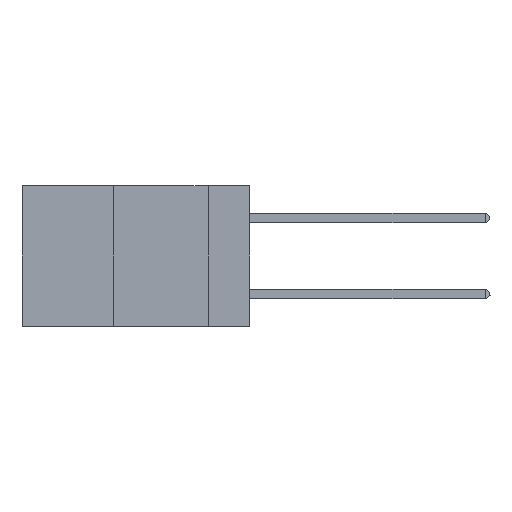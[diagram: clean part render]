
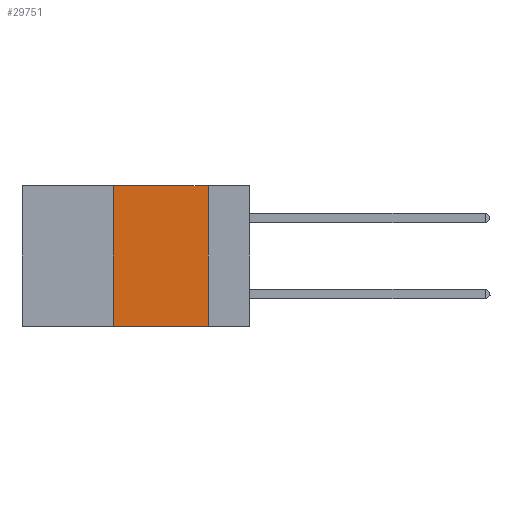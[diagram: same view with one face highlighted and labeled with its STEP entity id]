
A CAD part, left-side view. The second image highlights one B-rep face of the part: STEP entity #29751.
In plain terms, the highlighted planar face has unit normal (-1, 0, 0).
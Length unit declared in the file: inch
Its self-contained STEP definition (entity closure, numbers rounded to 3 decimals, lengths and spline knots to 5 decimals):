
#1965 = ORIENTED_EDGE ( 'NONE', *, *, #23945, .F. ) ;
#4214 = CARTESIAN_POINT ( 'NONE',  ( 0., 0.36, 0. ) ) ;
#5180 = PLANE ( 'NONE',  #34806 ) ;
#7371 = CARTESIAN_POINT ( 'NONE',  ( 0., 0.36, 0. ) ) ;
#8310 = ORIENTED_EDGE ( 'NONE', *, *, #18943, .T. ) ;
#10808 = VECTOR ( 'NONE', #39296, 39.37008 ) ;
#13116 = CARTESIAN_POINT ( 'NONE',  ( 0., 0.11, 0. ) ) ;
#13120 = VERTEX_POINT ( 'NONE', #23907 ) ;
#13730 = DIRECTION ( 'NONE',  ( 0., -1., 0. ) ) ;
#14348 = EDGE_CURVE ( 'NONE', #31260, #37553, #38616, .T. ) ;
#16620 = DIRECTION ( 'NONE',  ( 0., 0., 1. ) ) ;
#18021 = CARTESIAN_POINT ( 'NONE',  ( 0., 0.36, -0.37 ) ) ;
#18943 = EDGE_CURVE ( 'NONE', #31260, #19917, #36037, .T. ) ;
#18962 = DIRECTION ( 'NONE',  ( 0., 0., -1. ) ) ;
#19917 = VERTEX_POINT ( 'NONE', #34206 ) ;
#23149 = CARTESIAN_POINT ( 'NONE',  ( 0., 0.6, -0.37 ) ) ;
#23907 = CARTESIAN_POINT ( 'NONE',  ( 0., 0.11, 0. ) ) ;
#23945 = EDGE_CURVE ( 'NONE', #37553, #13120, #39540, .T. ) ;
#24245 = CARTESIAN_POINT ( 'NONE',  ( 0., 0.6, 0. ) ) ;
#24511 = DIRECTION ( 'NONE',  ( 1., 0., 0. ) ) ;
#24743 = VECTOR ( 'NONE', #13730, 39.37008 ) ;
#25908 = EDGE_LOOP ( 'NONE', ( #38144, #1965, #29895, #8310 ) ) ;
#26432 = VECTOR ( 'NONE', #18962, 39.37008 ) ;
#26715 = EDGE_CURVE ( 'NONE', #13120, #19917, #27940, .T. ) ;
#27940 = LINE ( 'NONE', #13116, #26432 ) ;
#29751 = ADVANCED_FACE ( 'NONE', ( #34858 ), #5180, .F. ) ;
#29895 = ORIENTED_EDGE ( 'NONE', *, *, #14348, .F. ) ;
#31260 = VERTEX_POINT ( 'NONE', #18021 ) ;
#32708 = CARTESIAN_POINT ( 'NONE',  ( 0., 0.6, 0. ) ) ;
#32761 = VECTOR ( 'NONE', #16620, 39.37008 ) ;
#34039 = DIRECTION ( 'NONE',  ( 0., 0., -1. ) ) ;
#34206 = CARTESIAN_POINT ( 'NONE',  ( 0., 0.11, -0.37 ) ) ;
#34806 = AXIS2_PLACEMENT_3D ( 'NONE', #24245, #24511, #34039 ) ;
#34858 = FACE_OUTER_BOUND ( 'NONE', #25908, .T. ) ;
#36037 = LINE ( 'NONE', #23149, #10808 ) ;
#37553 = VERTEX_POINT ( 'NONE', #7371 ) ;
#38144 = ORIENTED_EDGE ( 'NONE', *, *, #26715, .F. ) ;
#38616 = LINE ( 'NONE', #4214, #32761 ) ;
#39296 = DIRECTION ( 'NONE',  ( 0., -1., 0. ) ) ;
#39540 = LINE ( 'NONE', #32708, #24743 ) ;
